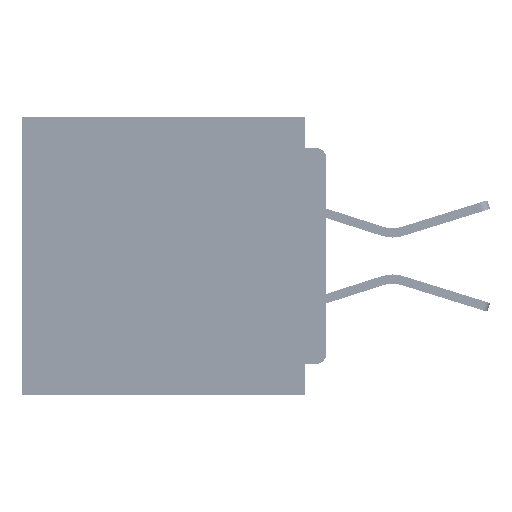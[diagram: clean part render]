
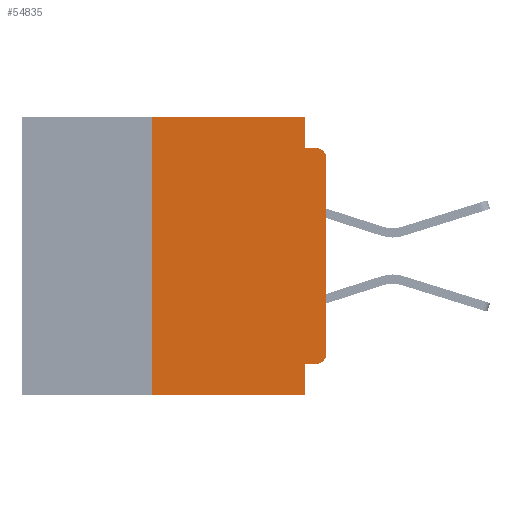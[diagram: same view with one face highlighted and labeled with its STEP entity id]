
A CAD part, left-side view. The second image highlights one B-rep face of the part: STEP entity #54835.
In plain terms, the highlighted planar face has unit normal (-1, 0, 0).
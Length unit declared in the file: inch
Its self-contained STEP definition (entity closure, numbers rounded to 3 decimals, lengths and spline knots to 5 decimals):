
#640 = VECTOR ( 'NONE', #12399, 39.37008 ) ;
#1340 = AXIS2_PLACEMENT_3D ( 'NONE', #11833, #49847, #17300 ) ;
#1765 = EDGE_CURVE ( 'NONE', #18613, #38490, #20954, .T. ) ;
#1866 = DIRECTION ( 'NONE',  ( 0., 0., -1. ) ) ;
#1880 = LINE ( 'NONE', #52189, #57984 ) ;
#2478 = AXIS2_PLACEMENT_3D ( 'NONE', #56039, #34391, #1866 ) ;
#2519 = VERTEX_POINT ( 'NONE', #19426 ) ;
#3009 = CARTESIAN_POINT ( 'NONE',  ( 0., 0.015, -0.045 ) ) ;
#3914 = EDGE_CURVE ( 'NONE', #68753, #58943, #18348, .T. ) ;
#4249 = ORIENTED_EDGE ( 'NONE', *, *, #3914, .F. ) ;
#9039 = LINE ( 'NONE', #67588, #65121 ) ;
#10052 = EDGE_CURVE ( 'NONE', #46439, #58943, #9039, .T. ) ;
#10160 = DIRECTION ( 'NONE',  ( 0., -1., 0. ) ) ;
#10619 = VECTOR ( 'NONE', #25226, 39.37008 ) ;
#11049 = EDGE_LOOP ( 'NONE', ( #25670, #44502, #34110, #68651, #57898, #22180, #25807, #4249, #42622, #26562 ) ) ;
#11110 = VECTOR ( 'NONE', #56457, 39.37008 ) ;
#11833 = CARTESIAN_POINT ( 'NONE',  ( 0., 0.015, -0.34 ) ) ;
#11945 = EDGE_CURVE ( 'NONE', #55872, #31208, #68892, .T. ) ;
#12399 = DIRECTION ( 'NONE',  ( 0., 0., 1. ) ) ;
#13769 = CARTESIAN_POINT ( 'NONE',  ( 0., 0., -0.355 ) ) ;
#14875 = EDGE_CURVE ( 'NONE', #31208, #38490, #40393, .T. ) ;
#15043 = LINE ( 'NONE', #28756, #640 ) ;
#15321 = CIRCLE ( 'NONE', #1340, 0.015 ) ;
#15877 = CARTESIAN_POINT ( 'NONE',  ( 0., 0.031, -0.045 ) ) ;
#15889 = EDGE_CURVE ( 'NONE', #30868, #68753, #29318, .T. ) ;
#17300 = DIRECTION ( 'NONE',  ( 0., 0., -1. ) ) ;
#18348 = LINE ( 'NONE', #19181, #34475 ) ;
#18451 = CARTESIAN_POINT ( 'NONE',  ( 0., 0.031, 0. ) ) ;
#18613 = VERTEX_POINT ( 'NONE', #53072 ) ;
#19181 = CARTESIAN_POINT ( 'NONE',  ( 0., 0.031, -0.4 ) ) ;
#19426 = CARTESIAN_POINT ( 'NONE',  ( 0., 0.25, 0. ) ) ;
#20954 = CIRCLE ( 'NONE', #42442, 0.015 ) ;
#20982 = DIRECTION ( 'NONE',  ( 0., 0., -1. ) ) ;
#22180 = ORIENTED_EDGE ( 'NONE', *, *, #31660, .F. ) ;
#25033 = LINE ( 'NONE', #57779, #10619 ) ;
#25226 = DIRECTION ( 'NONE',  ( 0., -1., 0. ) ) ;
#25670 = ORIENTED_EDGE ( 'NONE', *, *, #58855, .T. ) ;
#25807 = ORIENTED_EDGE ( 'NONE', *, *, #10052, .T. ) ;
#26562 = ORIENTED_EDGE ( 'NONE', *, *, #33434, .T. ) ;
#26609 = CARTESIAN_POINT ( 'NONE',  ( 0., 0.031, -0.355 ) ) ;
#28756 = CARTESIAN_POINT ( 'NONE',  ( 0., 0., 0. ) ) ;
#29318 = LINE ( 'NONE', #13769, #54816 ) ;
#30868 = VERTEX_POINT ( 'NONE', #56101 ) ;
#31208 = VERTEX_POINT ( 'NONE', #15877 ) ;
#31660 = EDGE_CURVE ( 'NONE', #46439, #2519, #1880, .T. ) ;
#33434 = EDGE_CURVE ( 'NONE', #30868, #57862, #15321, .T. ) ;
#34110 = ORIENTED_EDGE ( 'NONE', *, *, #14875, .F. ) ;
#34391 = DIRECTION ( 'NONE',  ( 1., 0., 0. ) ) ;
#34475 = VECTOR ( 'NONE', #20982, 39.37008 ) ;
#35004 = DIRECTION ( 'NONE',  ( 0., -1., 0. ) ) ;
#37158 = CARTESIAN_POINT ( 'NONE',  ( 0., 0., -0.045 ) ) ;
#37792 = CARTESIAN_POINT ( 'NONE',  ( 0., 0.031, 0. ) ) ;
#38490 = VERTEX_POINT ( 'NONE', #3009 ) ;
#38691 = VECTOR ( 'NONE', #10160, 39.37008 ) ;
#40393 = LINE ( 'NONE', #37158, #38691 ) ;
#42442 = AXIS2_PLACEMENT_3D ( 'NONE', #62759, #62678, #62696 ) ;
#42622 = ORIENTED_EDGE ( 'NONE', *, *, #15889, .F. ) ;
#44502 = ORIENTED_EDGE ( 'NONE', *, *, #1765, .T. ) ;
#46307 = DIRECTION ( 'NONE',  ( 0., 1., 0. ) ) ;
#46439 = VERTEX_POINT ( 'NONE', #46521 ) ;
#46521 = CARTESIAN_POINT ( 'NONE',  ( 0., 0.25, -0.4 ) ) ;
#46743 = DIRECTION ( 'NONE',  ( 0., 0., 1. ) ) ;
#49847 = DIRECTION ( 'NONE',  ( -1., 0., 0. ) ) ;
#51323 = CARTESIAN_POINT ( 'NONE',  ( 0., 0.031, -0.4 ) ) ;
#52152 = CARTESIAN_POINT ( 'NONE',  ( 0., 0., -0.34 ) ) ;
#52189 = CARTESIAN_POINT ( 'NONE',  ( 0., 0.25, -0.4 ) ) ;
#53072 = CARTESIAN_POINT ( 'NONE',  ( 0., 0., -0.06 ) ) ;
#54816 = VECTOR ( 'NONE', #46307, 39.37008 ) ;
#54835 = ADVANCED_FACE ( 'NONE', ( #56940 ), #66962, .F. ) ;
#55872 = VERTEX_POINT ( 'NONE', #37792 ) ;
#56039 = CARTESIAN_POINT ( 'NONE',  ( 0., 0.437, 0. ) ) ;
#56101 = CARTESIAN_POINT ( 'NONE',  ( 0., 0.015, -0.355 ) ) ;
#56457 = DIRECTION ( 'NONE',  ( 0., 0., -1. ) ) ;
#56940 = FACE_OUTER_BOUND ( 'NONE', #11049, .T. ) ;
#57779 = CARTESIAN_POINT ( 'NONE',  ( 0., 0.437, 0. ) ) ;
#57862 = VERTEX_POINT ( 'NONE', #52152 ) ;
#57898 = ORIENTED_EDGE ( 'NONE', *, *, #58423, .F. ) ;
#57984 = VECTOR ( 'NONE', #46743, 39.37008 ) ;
#58423 = EDGE_CURVE ( 'NONE', #2519, #55872, #25033, .T. ) ;
#58855 = EDGE_CURVE ( 'NONE', #57862, #18613, #15043, .T. ) ;
#58943 = VERTEX_POINT ( 'NONE', #51323 ) ;
#62678 = DIRECTION ( 'NONE',  ( -1., 0., 0. ) ) ;
#62696 = DIRECTION ( 'NONE',  ( 0., 0., -1. ) ) ;
#62759 = CARTESIAN_POINT ( 'NONE',  ( 0., 0.015, -0.06 ) ) ;
#65121 = VECTOR ( 'NONE', #35004, 39.37008 ) ;
#66962 = PLANE ( 'NONE',  #2478 ) ;
#67588 = CARTESIAN_POINT ( 'NONE',  ( 0., 0.437, -0.4 ) ) ;
#68651 = ORIENTED_EDGE ( 'NONE', *, *, #11945, .F. ) ;
#68753 = VERTEX_POINT ( 'NONE', #26609 ) ;
#68892 = LINE ( 'NONE', #18451, #11110 ) ;
